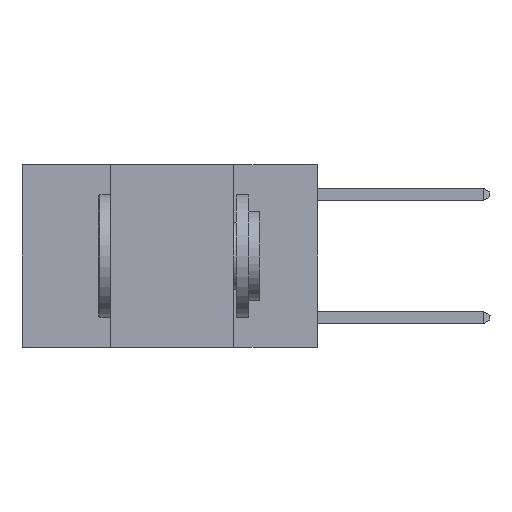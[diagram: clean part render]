
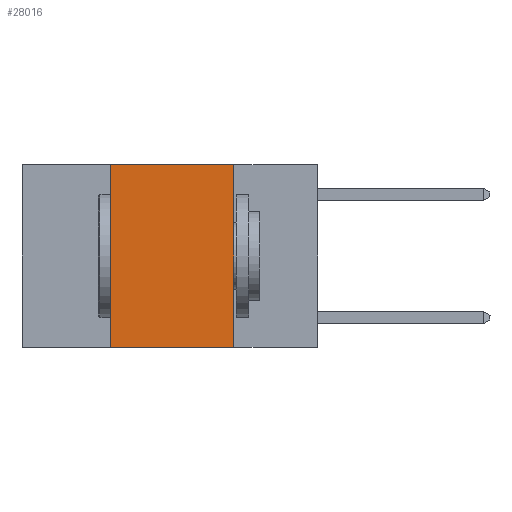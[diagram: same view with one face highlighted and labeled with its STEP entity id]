
A CAD part, left-side view. The second image highlights one B-rep face of the part: STEP entity #28016.
In plain terms, the highlighted planar face has unit normal (-1, 0, 0).
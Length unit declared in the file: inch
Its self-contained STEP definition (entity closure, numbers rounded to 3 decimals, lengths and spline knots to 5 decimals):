
#434 = CARTESIAN_POINT ( 'NONE',  ( 0., 0.17, 0. ) ) ;
#1096 = DIRECTION ( 'NONE',  ( 0., 0., -1. ) ) ;
#1992 = CARTESIAN_POINT ( 'NONE',  ( 0., 0.6, 0. ) ) ;
#3071 = CARTESIAN_POINT ( 'NONE',  ( 0., 0.6, 0. ) ) ;
#4532 = CARTESIAN_POINT ( 'NONE',  ( 0., 0.6, -0.37 ) ) ;
#4663 = EDGE_LOOP ( 'NONE', ( #19159, #28450, #23075, #12625 ) ) ;
#6693 = EDGE_CURVE ( 'NONE', #10343, #21273, #24660, .T. ) ;
#7598 = LINE ( 'NONE', #434, #20511 ) ;
#9038 = CARTESIAN_POINT ( 'NONE',  ( 0., 0.17, -0.37 ) ) ;
#9737 = VECTOR ( 'NONE', #13199, 39.37008 ) ;
#10343 = VERTEX_POINT ( 'NONE', #14829 ) ;
#11787 = FACE_OUTER_BOUND ( 'NONE', #4663, .T. ) ;
#12625 = ORIENTED_EDGE ( 'NONE', *, *, #6693, .T. ) ;
#12800 = EDGE_CURVE ( 'NONE', #26004, #21273, #7598, .T. ) ;
#13199 = DIRECTION ( 'NONE',  ( 0., -1., 0. ) ) ;
#13215 = EDGE_CURVE ( 'NONE', #10343, #31867, #25466, .T. ) ;
#13864 = AXIS2_PLACEMENT_3D ( 'NONE', #1992, #29731, #17125 ) ;
#13981 = LINE ( 'NONE', #3071, #9737 ) ;
#14829 = CARTESIAN_POINT ( 'NONE',  ( 0., 0.42, -0.37 ) ) ;
#15033 = CARTESIAN_POINT ( 'NONE',  ( 0., 0.42, 0. ) ) ;
#15663 = DIRECTION ( 'NONE',  ( 0., 0., 1. ) ) ;
#17125 = DIRECTION ( 'NONE',  ( 0., 0., -1. ) ) ;
#19159 = ORIENTED_EDGE ( 'NONE', *, *, #12800, .F. ) ;
#20511 = VECTOR ( 'NONE', #1096, 39.37008 ) ;
#21273 = VERTEX_POINT ( 'NONE', #9038 ) ;
#21942 = PLANE ( 'NONE',  #13864 ) ;
#22988 = CARTESIAN_POINT ( 'NONE',  ( 0., 0.42, 0. ) ) ;
#23075 = ORIENTED_EDGE ( 'NONE', *, *, #13215, .F. ) ;
#23511 = CARTESIAN_POINT ( 'NONE',  ( 0., 0.17, 0. ) ) ;
#24235 = VECTOR ( 'NONE', #15663, 39.37008 ) ;
#24660 = LINE ( 'NONE', #4532, #27452 ) ;
#25466 = LINE ( 'NONE', #22988, #24235 ) ;
#26004 = VERTEX_POINT ( 'NONE', #23511 ) ;
#27452 = VECTOR ( 'NONE', #31937, 39.37008 ) ;
#28016 = ADVANCED_FACE ( 'NONE', ( #11787 ), #21942, .F. ) ;
#28450 = ORIENTED_EDGE ( 'NONE', *, *, #32303, .F. ) ;
#29731 = DIRECTION ( 'NONE',  ( 1., 0., 0. ) ) ;
#31867 = VERTEX_POINT ( 'NONE', #15033 ) ;
#31937 = DIRECTION ( 'NONE',  ( 0., -1., 0. ) ) ;
#32303 = EDGE_CURVE ( 'NONE', #31867, #26004, #13981, .T. ) ;
